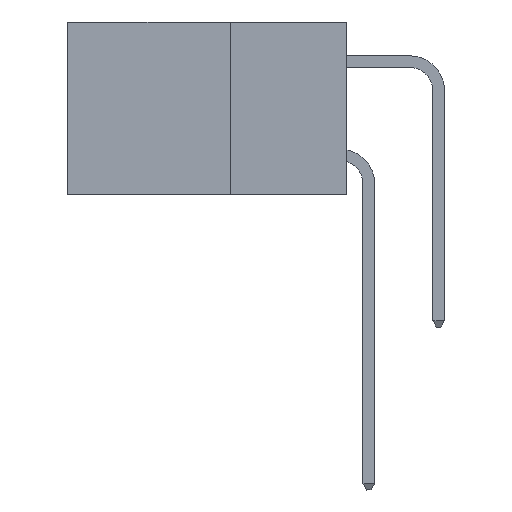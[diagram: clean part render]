
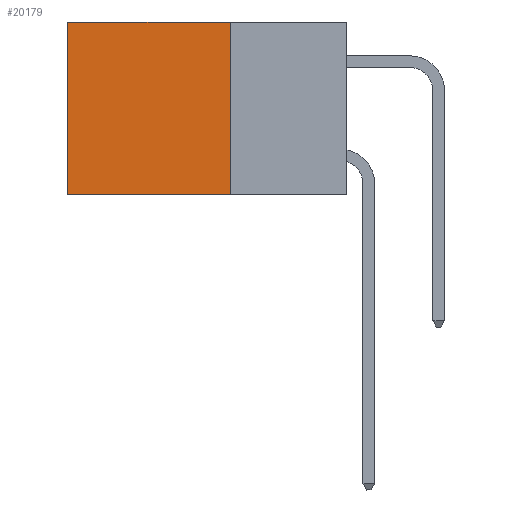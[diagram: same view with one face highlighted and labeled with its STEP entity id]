
A CAD part, left-side view. The second image highlights one B-rep face of the part: STEP entity #20179.
In plain terms, the highlighted planar face has unit normal (-1, 0, 0).
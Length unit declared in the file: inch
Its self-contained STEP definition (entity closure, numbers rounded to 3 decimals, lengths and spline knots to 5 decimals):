
#1419 = VECTOR ( 'NONE', #18437, 39.37008 ) ;
#2254 = AXIS2_PLACEMENT_3D ( 'NONE', #5917, #4099, #17468 ) ;
#3112 = FACE_OUTER_BOUND ( 'NONE', #10342, .T. ) ;
#3759 = PLANE ( 'NONE',  #2254 ) ;
#3896 = ORIENTED_EDGE ( 'NONE', *, *, #24426, .F. ) ;
#3998 = LINE ( 'NONE', #8718, #17486 ) ;
#4099 = DIRECTION ( 'NONE',  ( 1., 0., 0. ) ) ;
#4835 = CARTESIAN_POINT ( 'NONE',  ( 0.2875, 0.25, 0. ) ) ;
#5236 = CARTESIAN_POINT ( 'NONE',  ( 0.2875, 0.6, 0. ) ) ;
#5917 = CARTESIAN_POINT ( 'NONE',  ( 0.2875, 0.25, 0. ) ) ;
#6031 = VERTEX_POINT ( 'NONE', #5236 ) ;
#6346 = VERTEX_POINT ( 'NONE', #4835 ) ;
#7041 = DIRECTION ( 'NONE',  ( 0., 1., 0. ) ) ;
#8718 = CARTESIAN_POINT ( 'NONE',  ( 0.2875, 0.25, 0. ) ) ;
#10286 = VECTOR ( 'NONE', #7041, 39.37008 ) ;
#10342 = EDGE_LOOP ( 'NONE', ( #14829, #3896, #12684, #22428 ) ) ;
#11530 = VERTEX_POINT ( 'NONE', #17070 ) ;
#12684 = ORIENTED_EDGE ( 'NONE', *, *, #13359, .F. ) ;
#13215 = DIRECTION ( 'NONE',  ( 0., 1., 0. ) ) ;
#13359 = EDGE_CURVE ( 'NONE', #6346, #11530, #3998, .T. ) ;
#13718 = LINE ( 'NONE', #16525, #1419 ) ;
#14829 = ORIENTED_EDGE ( 'NONE', *, *, #22889, .T. ) ;
#16386 = VECTOR ( 'NONE', #13215, 39.37008 ) ;
#16525 = CARTESIAN_POINT ( 'NONE',  ( 0.2875, 0.6, 0. ) ) ;
#17070 = CARTESIAN_POINT ( 'NONE',  ( 0.2875, 0.25, -0.37 ) ) ;
#17344 = VERTEX_POINT ( 'NONE', #22312 ) ;
#17468 = DIRECTION ( 'NONE',  ( 0., 0., -1. ) ) ;
#17486 = VECTOR ( 'NONE', #18216, 39.37008 ) ;
#18216 = DIRECTION ( 'NONE',  ( 0., 0., -1. ) ) ;
#18437 = DIRECTION ( 'NONE',  ( 0., 0., -1. ) ) ;
#18854 = EDGE_CURVE ( 'NONE', #6346, #6031, #19755, .T. ) ;
#19755 = LINE ( 'NONE', #20579, #16386 ) ;
#20084 = LINE ( 'NONE', #22707, #10286 ) ;
#20179 = ADVANCED_FACE ( 'NONE', ( #3112 ), #3759, .F. ) ;
#20579 = CARTESIAN_POINT ( 'NONE',  ( 0.2875, 0.25, 0. ) ) ;
#22312 = CARTESIAN_POINT ( 'NONE',  ( 0.2875, 0.6, -0.37 ) ) ;
#22428 = ORIENTED_EDGE ( 'NONE', *, *, #18854, .T. ) ;
#22707 = CARTESIAN_POINT ( 'NONE',  ( 0.2875, 0.25, -0.37 ) ) ;
#22889 = EDGE_CURVE ( 'NONE', #6031, #17344, #13718, .T. ) ;
#24426 = EDGE_CURVE ( 'NONE', #11530, #17344, #20084, .T. ) ;
